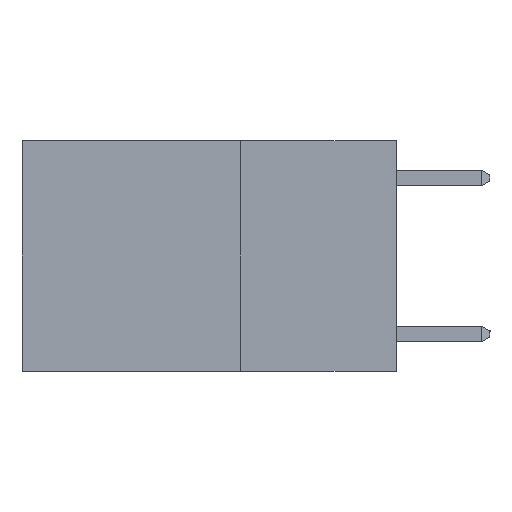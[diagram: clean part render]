
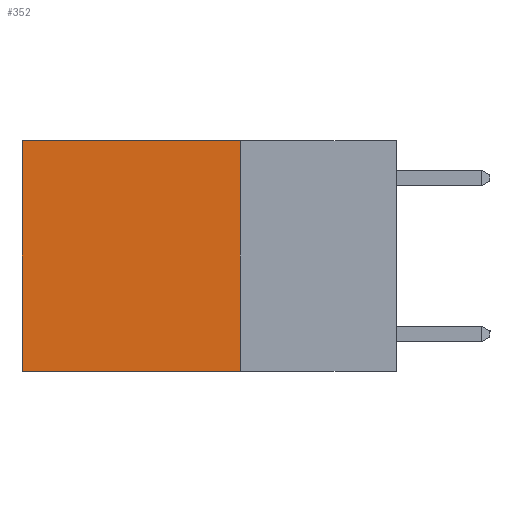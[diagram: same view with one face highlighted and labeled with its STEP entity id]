
A CAD part, left-side view. The second image highlights one B-rep face of the part: STEP entity #352.
In plain terms, the highlighted planar face has unit normal (-1, 0, 0).
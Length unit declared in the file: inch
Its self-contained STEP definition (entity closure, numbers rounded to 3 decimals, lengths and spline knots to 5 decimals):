
#83 = DIRECTION ( 'NONE',  ( 0., 0., -1. ) ) ;
#352 = ADVANCED_FACE ( 'NONE', ( #5931 ), #10936, .F. ) ;
#741 = CARTESIAN_POINT ( 'NONE',  ( 0.2625, 0.25, -0.37 ) ) ;
#978 = AXIS2_PLACEMENT_3D ( 'NONE', #1560, #6700, #83 ) ;
#1368 = EDGE_CURVE ( 'NONE', #2789, #8338, #8054, .T. ) ;
#1560 = CARTESIAN_POINT ( 'NONE',  ( 0.2625, 0.25, 0. ) ) ;
#1662 = DIRECTION ( 'NONE',  ( 0., 1., 0. ) ) ;
#1787 = DIRECTION ( 'NONE',  ( 0., 0., -1. ) ) ;
#2284 = VECTOR ( 'NONE', #3151, 39.37008 ) ;
#2319 = CARTESIAN_POINT ( 'NONE',  ( 0.2625, 0.6, 0. ) ) ;
#2789 = VERTEX_POINT ( 'NONE', #7355 ) ;
#2794 = EDGE_CURVE ( 'NONE', #5381, #5211, #10336, .T. ) ;
#2977 = EDGE_CURVE ( 'NONE', #2789, #5381, #10993, .T. ) ;
#3075 = ORIENTED_EDGE ( 'NONE', *, *, #9604, .F. ) ;
#3151 = DIRECTION ( 'NONE',  ( 0., 0., -1. ) ) ;
#4344 = CARTESIAN_POINT ( 'NONE',  ( 0.2625, 0.25, 0. ) ) ;
#4389 = VECTOR ( 'NONE', #1662, 39.37008 ) ;
#4822 = DIRECTION ( 'NONE',  ( 0., 1., 0. ) ) ;
#4836 = ORIENTED_EDGE ( 'NONE', *, *, #2977, .T. ) ;
#5211 = VERTEX_POINT ( 'NONE', #10981 ) ;
#5366 = VECTOR ( 'NONE', #1787, 39.37008 ) ;
#5381 = VERTEX_POINT ( 'NONE', #8698 ) ;
#5931 = FACE_OUTER_BOUND ( 'NONE', #7989, .T. ) ;
#6700 = DIRECTION ( 'NONE',  ( 1., 0., 0. ) ) ;
#7308 = ORIENTED_EDGE ( 'NONE', *, *, #2794, .T. ) ;
#7355 = CARTESIAN_POINT ( 'NONE',  ( 0.2625, 0.25, 0. ) ) ;
#7685 = ORIENTED_EDGE ( 'NONE', *, *, #1368, .F. ) ;
#7989 = EDGE_LOOP ( 'NONE', ( #7308, #3075, #7685, #4836 ) ) ;
#8025 = VECTOR ( 'NONE', #4822, 39.37008 ) ;
#8054 = LINE ( 'NONE', #4344, #5366 ) ;
#8272 = LINE ( 'NONE', #8933, #8025 ) ;
#8338 = VERTEX_POINT ( 'NONE', #741 ) ;
#8698 = CARTESIAN_POINT ( 'NONE',  ( 0.2625, 0.6, 0. ) ) ;
#8933 = CARTESIAN_POINT ( 'NONE',  ( 0.2625, 0.25, -0.37 ) ) ;
#9604 = EDGE_CURVE ( 'NONE', #8338, #5211, #8272, .T. ) ;
#9983 = CARTESIAN_POINT ( 'NONE',  ( 0.2625, 0.25, 0. ) ) ;
#10336 = LINE ( 'NONE', #2319, #2284 ) ;
#10936 = PLANE ( 'NONE',  #978 ) ;
#10981 = CARTESIAN_POINT ( 'NONE',  ( 0.2625, 0.6, -0.37 ) ) ;
#10993 = LINE ( 'NONE', #9983, #4389 ) ;
